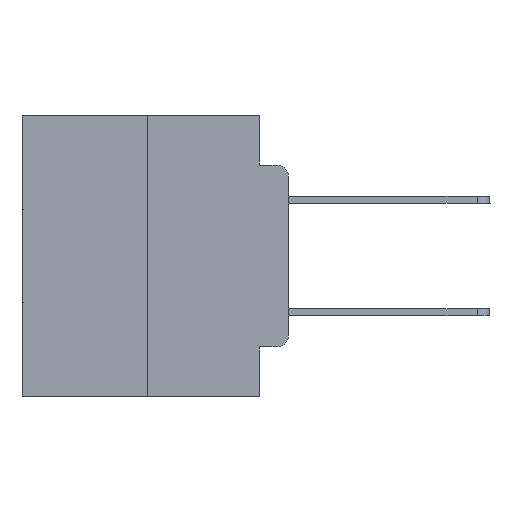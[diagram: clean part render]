
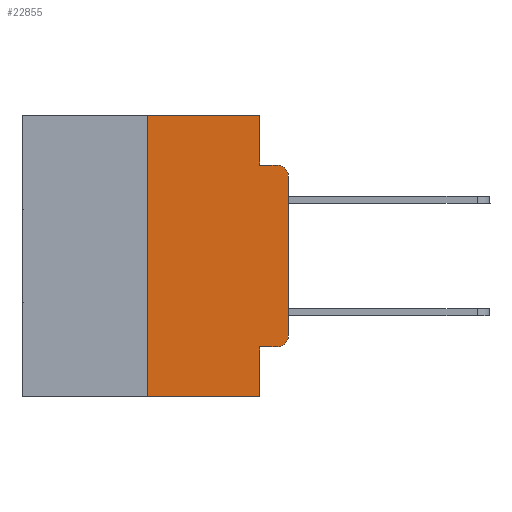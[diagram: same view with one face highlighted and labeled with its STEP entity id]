
A CAD part, left-side view. The second image highlights one B-rep face of the part: STEP entity #22855.
In plain terms, the highlighted planar face has unit normal (-1, 0, 0).
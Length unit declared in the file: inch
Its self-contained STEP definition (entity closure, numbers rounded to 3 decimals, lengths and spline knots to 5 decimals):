
#80 = CIRCLE ( 'NONE', #3386, 0.02 ) ;
#404 = DIRECTION ( 'NONE',  ( 1., 0., 0. ) ) ;
#506 = AXIS2_PLACEMENT_3D ( 'NONE', #19117, #27392, #3675 ) ;
#611 = CARTESIAN_POINT ( 'NONE',  ( 0., 0.25, -0.5 ) ) ;
#1079 = AXIS2_PLACEMENT_3D ( 'NONE', #21881, #404, #17417 ) ;
#1228 = CARTESIAN_POINT ( 'NONE',  ( 0., 0.02, -0.0885 ) ) ;
#1689 = LINE ( 'NONE', #10686, #26821 ) ;
#2240 = PLANE ( 'NONE',  #1079 ) ;
#2539 = VECTOR ( 'NONE', #7699, 39.37008 ) ;
#2556 = ORIENTED_EDGE ( 'NONE', *, *, #20834, .T. ) ;
#2762 = EDGE_CURVE ( 'NONE', #9349, #23461, #1689, .T. ) ;
#3156 = EDGE_CURVE ( 'NONE', #27679, #20098, #4724, .T. ) ;
#3386 = AXIS2_PLACEMENT_3D ( 'NONE', #21471, #12892, #8241 ) ;
#3593 = CARTESIAN_POINT ( 'NONE',  ( 0., 0.051, -0.5 ) ) ;
#3675 = DIRECTION ( 'NONE',  ( 0., 0., -1. ) ) ;
#3959 = ORIENTED_EDGE ( 'NONE', *, *, #11988, .F. ) ;
#4305 = DIRECTION ( 'NONE',  ( 0., 0., 1. ) ) ;
#4644 = DIRECTION ( 'NONE',  ( 0., 0., -1. ) ) ;
#4724 = LINE ( 'NONE', #18823, #27466 ) ;
#4793 = EDGE_CURVE ( 'NONE', #9349, #11428, #19039, .T. ) ;
#6880 = LINE ( 'NONE', #9216, #15402 ) ;
#7699 = DIRECTION ( 'NONE',  ( 0., 0., 1. ) ) ;
#8241 = DIRECTION ( 'NONE',  ( 0., 0., -1. ) ) ;
#8565 = VERTEX_POINT ( 'NONE', #11346 ) ;
#8684 = EDGE_CURVE ( 'NONE', #27679, #11428, #27688, .T. ) ;
#9004 = CARTESIAN_POINT ( 'NONE',  ( 0., 0.051, 0. ) ) ;
#9195 = ORIENTED_EDGE ( 'NONE', *, *, #9564, .T. ) ;
#9216 = CARTESIAN_POINT ( 'NONE',  ( 0., 0.051, -0.0885 ) ) ;
#9349 = VERTEX_POINT ( 'NONE', #9692 ) ;
#9564 = EDGE_CURVE ( 'NONE', #16842, #26068, #20873, .T. ) ;
#9657 = VECTOR ( 'NONE', #13815, 39.37008 ) ;
#9692 = CARTESIAN_POINT ( 'NONE',  ( 0., 0.051, -0.4115 ) ) ;
#9704 = LINE ( 'NONE', #9004, #17212 ) ;
#9824 = EDGE_CURVE ( 'NONE', #19434, #10043, #6880, .T. ) ;
#9873 = CARTESIAN_POINT ( 'NONE',  ( 0., 0.051, -0.0885 ) ) ;
#10043 = VERTEX_POINT ( 'NONE', #1228 ) ;
#10141 = EDGE_CURVE ( 'NONE', #26068, #10043, #80, .T. ) ;
#10682 = ORIENTED_EDGE ( 'NONE', *, *, #10141, .T. ) ;
#10686 = CARTESIAN_POINT ( 'NONE',  ( 0., 0.051, -0.4115 ) ) ;
#11182 = ORIENTED_EDGE ( 'NONE', *, *, #3156, .F. ) ;
#11273 = CARTESIAN_POINT ( 'NONE',  ( 0., 0.02, -0.4115 ) ) ;
#11346 = CARTESIAN_POINT ( 'NONE',  ( 0., 0.051, 0. ) ) ;
#11428 = VERTEX_POINT ( 'NONE', #3593 ) ;
#11520 = CARTESIAN_POINT ( 'NONE',  ( 0., 0.473, -0.5 ) ) ;
#11604 = CARTESIAN_POINT ( 'NONE',  ( 0., 0.473, 0. ) ) ;
#11634 = DIRECTION ( 'NONE',  ( 0., 0., -1. ) ) ;
#11988 = EDGE_CURVE ( 'NONE', #20098, #8565, #25052, .T. ) ;
#12577 = VECTOR ( 'NONE', #11634, 39.37008 ) ;
#12892 = DIRECTION ( 'NONE',  ( -1., 0., 0. ) ) ;
#13364 = CARTESIAN_POINT ( 'NONE',  ( 0., 0., -0.3915 ) ) ;
#13671 = CIRCLE ( 'NONE', #506, 0.02 ) ;
#13807 = DIRECTION ( 'NONE',  ( 0., -1., 0. ) ) ;
#13815 = DIRECTION ( 'NONE',  ( 0., -1., 0. ) ) ;
#15402 = VECTOR ( 'NONE', #15686, 39.37008 ) ;
#15686 = DIRECTION ( 'NONE',  ( 0., -1., 0. ) ) ;
#15980 = ORIENTED_EDGE ( 'NONE', *, *, #25831, .F. ) ;
#16283 = FACE_OUTER_BOUND ( 'NONE', #27807, .T. ) ;
#16458 = ORIENTED_EDGE ( 'NONE', *, *, #8684, .T. ) ;
#16842 = VERTEX_POINT ( 'NONE', #13364 ) ;
#17212 = VECTOR ( 'NONE', #4644, 39.37008 ) ;
#17417 = DIRECTION ( 'NONE',  ( 0., 0., -1. ) ) ;
#18502 = ORIENTED_EDGE ( 'NONE', *, *, #9824, .F. ) ;
#18531 = CARTESIAN_POINT ( 'NONE',  ( 0., 0., 0. ) ) ;
#18823 = CARTESIAN_POINT ( 'NONE',  ( 0., 0.25, 0. ) ) ;
#18889 = ORIENTED_EDGE ( 'NONE', *, *, #4793, .F. ) ;
#19039 = LINE ( 'NONE', #26585, #12577 ) ;
#19117 = CARTESIAN_POINT ( 'NONE',  ( 0., 0.02, -0.3915 ) ) ;
#19434 = VERTEX_POINT ( 'NONE', #9873 ) ;
#19658 = VECTOR ( 'NONE', #13807, 39.37008 ) ;
#20098 = VERTEX_POINT ( 'NONE', #25513 ) ;
#20834 = EDGE_CURVE ( 'NONE', #23461, #16842, #13671, .T. ) ;
#20873 = LINE ( 'NONE', #18531, #2539 ) ;
#21471 = CARTESIAN_POINT ( 'NONE',  ( 0., 0.02, -0.1085 ) ) ;
#21881 = CARTESIAN_POINT ( 'NONE',  ( 0., 0.473, 0. ) ) ;
#22855 = ADVANCED_FACE ( 'NONE', ( #16283 ), #2240, .F. ) ;
#22931 = CARTESIAN_POINT ( 'NONE',  ( 0., 0., -0.1085 ) ) ;
#23461 = VERTEX_POINT ( 'NONE', #11273 ) ;
#25052 = LINE ( 'NONE', #11604, #19658 ) ;
#25513 = CARTESIAN_POINT ( 'NONE',  ( 0., 0.25, 0. ) ) ;
#25831 = EDGE_CURVE ( 'NONE', #8565, #19434, #9704, .T. ) ;
#25897 = DIRECTION ( 'NONE',  ( 0., -1., 0. ) ) ;
#26068 = VERTEX_POINT ( 'NONE', #22931 ) ;
#26585 = CARTESIAN_POINT ( 'NONE',  ( 0., 0.051, 0. ) ) ;
#26821 = VECTOR ( 'NONE', #25897, 39.37008 ) ;
#27392 = DIRECTION ( 'NONE',  ( -1., 0., 0. ) ) ;
#27466 = VECTOR ( 'NONE', #4305, 39.37008 ) ;
#27679 = VERTEX_POINT ( 'NONE', #611 ) ;
#27688 = LINE ( 'NONE', #11520, #9657 ) ;
#27807 = EDGE_LOOP ( 'NONE', ( #9195, #10682, #18502, #15980, #3959, #11182, #16458, #18889, #28046, #2556 ) ) ;
#28046 = ORIENTED_EDGE ( 'NONE', *, *, #2762, .T. ) ;
